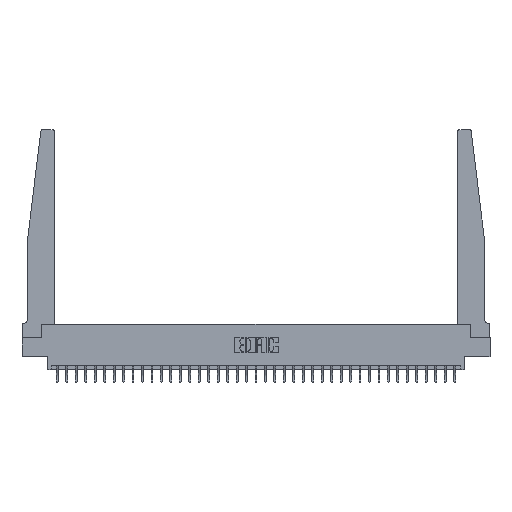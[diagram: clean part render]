
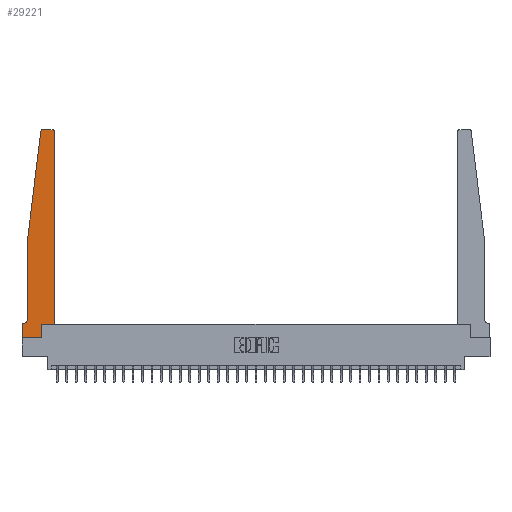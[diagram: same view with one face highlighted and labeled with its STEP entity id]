
A CAD part, top view. The second image highlights one B-rep face of the part: STEP entity #29221.
In plain terms, the highlighted planar face has unit normal (0, 0, 1).
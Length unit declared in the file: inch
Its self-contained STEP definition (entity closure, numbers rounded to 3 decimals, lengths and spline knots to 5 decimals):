
#345 = EDGE_CURVE ( 'NONE', #2525, #17342, #1192, .T. ) ;
#640 = AXIS2_PLACEMENT_3D ( 'NONE', #6969, #12715, #12542 ) ;
#1192 = CIRCLE ( 'NONE', #640, 0.05 ) ;
#1319 = CARTESIAN_POINT ( 'NONE',  ( 0.24675, 2.72367, 0.37 ) ) ;
#1490 = CARTESIAN_POINT ( 'NONE',  ( 0.425, 0.18, 0.37 ) ) ;
#1555 = DIRECTION ( 'NONE',  ( 1., 0., 0. ) ) ;
#2019 = VERTEX_POINT ( 'NONE', #26142 ) ;
#2291 = AXIS2_PLACEMENT_3D ( 'NONE', #24338, #11249, #11412 ) ;
#2525 = VERTEX_POINT ( 'NONE', #8610 ) ;
#3026 = LINE ( 'NONE', #28968, #8083 ) ;
#3431 = EDGE_CURVE ( 'NONE', #5119, #8361, #30140, .T. ) ;
#3450 = DIRECTION ( 'NONE',  ( 1., 0., 0. ) ) ;
#3470 = VERTEX_POINT ( 'NONE', #22153 ) ;
#3760 = EDGE_LOOP ( 'NONE', ( #4502, #13385, #6549, #25978, #32253, #25248, #10378, #16612, #12882, #30168, #9746, #25448 ) ) ;
#3975 = VECTOR ( 'NONE', #9419, 39.37008 ) ;
#4399 = FACE_OUTER_BOUND ( 'NONE', #3760, .T. ) ;
#4502 = ORIENTED_EDGE ( 'NONE', *, *, #3431, .T. ) ;
#5119 = VERTEX_POINT ( 'NONE', #8600 ) ;
#5509 = CIRCLE ( 'NONE', #2291, 0.03 ) ;
#5583 = EDGE_CURVE ( 'NONE', #3470, #8263, #18866, .T. ) ;
#5793 = CARTESIAN_POINT ( 'NONE',  ( 0., 0., 0.37 ) ) ;
#6285 = DIRECTION ( 'NONE',  ( 0., 0., 1. ) ) ;
#6380 = LINE ( 'NONE', #1490, #16459 ) ;
#6480 = CARTESIAN_POINT ( 'NONE',  ( 0.065, 0.1875, 0.37 ) ) ;
#6549 = ORIENTED_EDGE ( 'NONE', *, *, #27119, .T. ) ;
#6969 = CARTESIAN_POINT ( 'NONE',  ( 0.015, 0.2375, 0.37 ) ) ;
#8083 = VECTOR ( 'NONE', #11120, 39.37008 ) ;
#8263 = VERTEX_POINT ( 'NONE', #20565 ) ;
#8361 = VERTEX_POINT ( 'NONE', #14975 ) ;
#8583 = DIRECTION ( 'NONE',  ( 0., 0., 1. ) ) ;
#8600 = CARTESIAN_POINT ( 'NONE',  ( 0.395, 2.75, 0.37 ) ) ;
#8610 = CARTESIAN_POINT ( 'NONE',  ( 0.065, 0.2375, 0.37 ) ) ;
#8876 = AXIS2_PLACEMENT_3D ( 'NONE', #14408, #6285, #1555 ) ;
#9193 = DIRECTION ( 'NONE',  ( -1., 0., 0. ) ) ;
#9419 = DIRECTION ( 'NONE',  ( -1., 0., 0. ) ) ;
#9691 = EDGE_CURVE ( 'NONE', #28295, #3470, #19867, .T. ) ;
#9746 = ORIENTED_EDGE ( 'NONE', *, *, #31424, .T. ) ;
#9759 = EDGE_CURVE ( 'NONE', #17342, #31059, #14766, .T. ) ;
#10148 = VECTOR ( 'NONE', #30266, 39.37008 ) ;
#10378 = ORIENTED_EDGE ( 'NONE', *, *, #12314, .T. ) ;
#10861 = LINE ( 'NONE', #5793, #30568 ) ;
#11048 = DIRECTION ( 'NONE',  ( 1., 0., 0. ) ) ;
#11120 = DIRECTION ( 'NONE',  ( 0., -1., 0. ) ) ;
#11249 = DIRECTION ( 'NONE',  ( 0., 0., 1. ) ) ;
#11393 = CARTESIAN_POINT ( 'NONE',  ( 0.2605, 0.18, 0.37 ) ) ;
#11412 = DIRECTION ( 'NONE',  ( 1., 0., 0. ) ) ;
#11736 = DIRECTION ( 'NONE',  ( 0., 1., 0. ) ) ;
#11953 = DIRECTION ( 'NONE',  ( 0., 1., 0. ) ) ;
#12314 = EDGE_CURVE ( 'NONE', #31059, #2019, #10861, .T. ) ;
#12383 = VECTOR ( 'NONE', #11736, 39.37008 ) ;
#12542 = DIRECTION ( 'NONE',  ( -1., 0., 0. ) ) ;
#12715 = DIRECTION ( 'NONE',  ( 0., 0., -1. ) ) ;
#12882 = ORIENTED_EDGE ( 'NONE', *, *, #9691, .T. ) ;
#12922 = EDGE_CURVE ( 'NONE', #19345, #2525, #3026, .T. ) ;
#13074 = DIRECTION ( 'NONE',  ( 0., -1., 0. ) ) ;
#13385 = ORIENTED_EDGE ( 'NONE', *, *, #17680, .T. ) ;
#14408 = CARTESIAN_POINT ( 'NONE',  ( 0., 0.1875, 0.37 ) ) ;
#14508 = CARTESIAN_POINT ( 'NONE',  ( 0.25, 2.75, 0.37 ) ) ;
#14766 = LINE ( 'NONE', #6480, #29796 ) ;
#14975 = CARTESIAN_POINT ( 'NONE',  ( 0.27653, 2.75, 0.37 ) ) ;
#15467 = CARTESIAN_POINT ( 'NONE',  ( 0.065, 1.25, 0.37 ) ) ;
#15843 = EDGE_CURVE ( 'NONE', #31591, #5119, #30348, .T. ) ;
#16459 = VECTOR ( 'NONE', #11953, 39.37008 ) ;
#16612 = ORIENTED_EDGE ( 'NONE', *, *, #19466, .T. ) ;
#17342 = VERTEX_POINT ( 'NONE', #29814 ) ;
#17533 = CARTESIAN_POINT ( 'NONE',  ( 0.425, 2.72, 0.37 ) ) ;
#17680 = EDGE_CURVE ( 'NONE', #8361, #25206, #5509, .T. ) ;
#17833 = CARTESIAN_POINT ( 'NONE',  ( 0.065, 1.25, 0.37 ) ) ;
#18253 = VECTOR ( 'NONE', #3450, 39.37008 ) ;
#18866 = LINE ( 'NONE', #27028, #18253 ) ;
#19345 = VERTEX_POINT ( 'NONE', #17833 ) ;
#19466 = EDGE_CURVE ( 'NONE', #2019, #28295, #29399, .T. ) ;
#19867 = LINE ( 'NONE', #11393, #12383 ) ;
#20565 = CARTESIAN_POINT ( 'NONE',  ( 0.425, 0.18, 0.37 ) ) ;
#20756 = VECTOR ( 'NONE', #11048, 39.37008 ) ;
#21886 = PLANE ( 'NONE',  #8876 ) ;
#22153 = CARTESIAN_POINT ( 'NONE',  ( 0.2605, 0.18, 0.37 ) ) ;
#23343 = CARTESIAN_POINT ( 'NONE',  ( 0.395, 2.72, 0.37 ) ) ;
#24299 = CARTESIAN_POINT ( 'NONE',  ( 0., 0., 0.37 ) ) ;
#24338 = CARTESIAN_POINT ( 'NONE',  ( 0.27653, 2.72, 0.37 ) ) ;
#25206 = VERTEX_POINT ( 'NONE', #1319 ) ;
#25248 = ORIENTED_EDGE ( 'NONE', *, *, #9759, .T. ) ;
#25448 = ORIENTED_EDGE ( 'NONE', *, *, #15843, .T. ) ;
#25978 = ORIENTED_EDGE ( 'NONE', *, *, #12922, .T. ) ;
#26142 = CARTESIAN_POINT ( 'NONE',  ( 0., 0., 0.37 ) ) ;
#27028 = CARTESIAN_POINT ( 'NONE',  ( 0.425, 0.18, 0.37 ) ) ;
#27119 = EDGE_CURVE ( 'NONE', #25206, #19345, #28053, .T. ) ;
#28053 = LINE ( 'NONE', #15467, #10148 ) ;
#28295 = VERTEX_POINT ( 'NONE', #32511 ) ;
#28968 = CARTESIAN_POINT ( 'NONE',  ( 0.065, 1.25, 0.37 ) ) ;
#29221 = ADVANCED_FACE ( 'NONE', ( #4399 ), #21886, .T. ) ;
#29292 = DIRECTION ( 'NONE',  ( 1., 0., 0. ) ) ;
#29399 = LINE ( 'NONE', #24299, #20756 ) ;
#29796 = VECTOR ( 'NONE', #9193, 39.37008 ) ;
#29814 = CARTESIAN_POINT ( 'NONE',  ( 0.015, 0.1875, 0.37 ) ) ;
#30140 = LINE ( 'NONE', #14508, #3975 ) ;
#30168 = ORIENTED_EDGE ( 'NONE', *, *, #5583, .T. ) ;
#30266 = DIRECTION ( 'NONE',  ( -0.122, -0.992, 0. ) ) ;
#30348 = CIRCLE ( 'NONE', #32541, 0.03 ) ;
#30500 = CARTESIAN_POINT ( 'NONE',  ( 0., 0.1875, 0.37 ) ) ;
#30568 = VECTOR ( 'NONE', #13074, 39.37008 ) ;
#31059 = VERTEX_POINT ( 'NONE', #30500 ) ;
#31424 = EDGE_CURVE ( 'NONE', #8263, #31591, #6380, .T. ) ;
#31591 = VERTEX_POINT ( 'NONE', #17533 ) ;
#32253 = ORIENTED_EDGE ( 'NONE', *, *, #345, .T. ) ;
#32511 = CARTESIAN_POINT ( 'NONE',  ( 0.2605, 0., 0.37 ) ) ;
#32541 = AXIS2_PLACEMENT_3D ( 'NONE', #23343, #8583, #29292 ) ;
